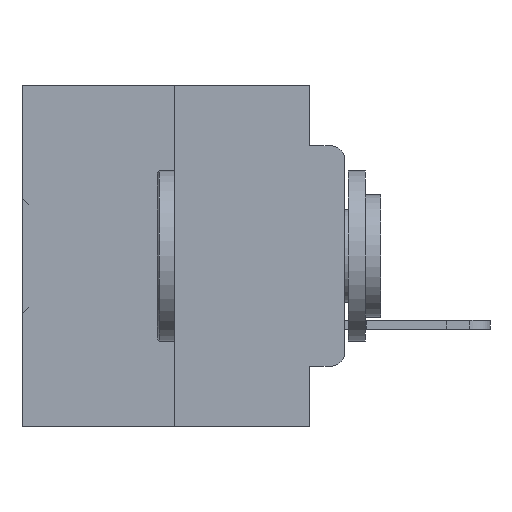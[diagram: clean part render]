
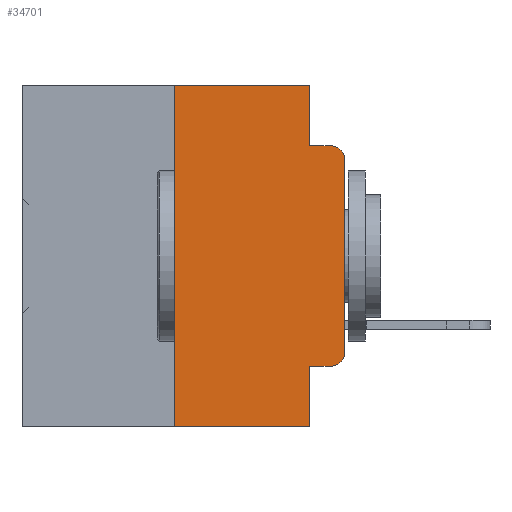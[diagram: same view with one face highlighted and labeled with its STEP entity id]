
A CAD part, left-side view. The second image highlights one B-rep face of the part: STEP entity #34701.
In plain terms, the highlighted planar face has unit normal (-1, 0, 0).
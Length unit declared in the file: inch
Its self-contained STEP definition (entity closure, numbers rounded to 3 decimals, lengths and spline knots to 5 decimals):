
#15 = CARTESIAN_POINT ( 'NONE',  ( 0., 0.051, 0. ) ) ;
#443 = EDGE_CURVE ( 'NONE', #1625, #14558, #28844, .T. ) ;
#584 = CARTESIAN_POINT ( 'NONE',  ( 0., 0.25, -0.5 ) ) ;
#693 = EDGE_CURVE ( 'NONE', #1318, #21653, #5347, .T. ) ;
#1136 = DIRECTION ( 'NONE',  ( 0., -1., 0. ) ) ;
#1315 = DIRECTION ( 'NONE',  ( 0., -1., 0. ) ) ;
#1318 = VERTEX_POINT ( 'NONE', #35348 ) ;
#1625 = VERTEX_POINT ( 'NONE', #584 ) ;
#2492 = AXIS2_PLACEMENT_3D ( 'NONE', #33372, #22013, #4564 ) ;
#2989 = CARTESIAN_POINT ( 'NONE',  ( 0., 0.051, -0.0885 ) ) ;
#3090 = VERTEX_POINT ( 'NONE', #33806 ) ;
#4260 = CARTESIAN_POINT ( 'NONE',  ( 0., 0.02, -0.0885 ) ) ;
#4564 = DIRECTION ( 'NONE',  ( 0., 0., -1. ) ) ;
#4862 = EDGE_LOOP ( 'NONE', ( #25022, #6470, #13825, #23275, #28598, #12962, #29947, #21050, #22870, #6101 ) ) ;
#5112 = DIRECTION ( 'NONE',  ( 0., 0., 1. ) ) ;
#5347 = CIRCLE ( 'NONE', #18586, 0.02 ) ;
#5638 = VERTEX_POINT ( 'NONE', #25015 ) ;
#5661 = VECTOR ( 'NONE', #1315, 39.37008 ) ;
#6101 = ORIENTED_EDGE ( 'NONE', *, *, #693, .T. ) ;
#6470 = ORIENTED_EDGE ( 'NONE', *, *, #9914, .T. ) ;
#6495 = DIRECTION ( 'NONE',  ( -1., 0., 0. ) ) ;
#6536 = VERTEX_POINT ( 'NONE', #15 ) ;
#7544 = AXIS2_PLACEMENT_3D ( 'NONE', #23849, #6495, #26697 ) ;
#8058 = CARTESIAN_POINT ( 'NONE',  ( 0., 0., 0. ) ) ;
#9769 = CARTESIAN_POINT ( 'NONE',  ( 0., 0.051, -0.4115 ) ) ;
#9914 = EDGE_CURVE ( 'NONE', #3090, #18468, #18216, .T. ) ;
#10889 = VECTOR ( 'NONE', #26927, 39.37008 ) ;
#11349 = EDGE_CURVE ( 'NONE', #11731, #26346, #11778, .T. ) ;
#11731 = VERTEX_POINT ( 'NONE', #26685 ) ;
#11777 = LINE ( 'NONE', #9769, #10889 ) ;
#11778 = LINE ( 'NONE', #13559, #26139 ) ;
#12584 = EDGE_CURVE ( 'NONE', #14558, #6536, #21103, .T. ) ;
#12962 = ORIENTED_EDGE ( 'NONE', *, *, #443, .F. ) ;
#13559 = CARTESIAN_POINT ( 'NONE',  ( 0., 0.051, 0. ) ) ;
#13646 = DIRECTION ( 'NONE',  ( 0., 0., 1. ) ) ;
#13825 = ORIENTED_EDGE ( 'NONE', *, *, #31699, .F. ) ;
#14158 = VECTOR ( 'NONE', #1136, 39.37008 ) ;
#14558 = VERTEX_POINT ( 'NONE', #20987 ) ;
#15344 = CARTESIAN_POINT ( 'NONE',  ( 0., 0.25, 0. ) ) ;
#18216 = CIRCLE ( 'NONE', #7544, 0.02 ) ;
#18345 = EDGE_CURVE ( 'NONE', #6536, #5638, #32594, .T. ) ;
#18468 = VERTEX_POINT ( 'NONE', #4260 ) ;
#18586 = AXIS2_PLACEMENT_3D ( 'NONE', #32917, #37445, #35901 ) ;
#18597 = CARTESIAN_POINT ( 'NONE',  ( 0., 0.051, -0.5 ) ) ;
#19162 = PLANE ( 'NONE',  #2492 ) ;
#20987 = CARTESIAN_POINT ( 'NONE',  ( 0., 0.25, 0. ) ) ;
#21050 = ORIENTED_EDGE ( 'NONE', *, *, #11349, .F. ) ;
#21103 = LINE ( 'NONE', #36110, #5661 ) ;
#21259 = VECTOR ( 'NONE', #13646, 39.37008 ) ;
#21653 = VERTEX_POINT ( 'NONE', #29732 ) ;
#21979 = VECTOR ( 'NONE', #5112, 39.37008 ) ;
#22013 = DIRECTION ( 'NONE',  ( 1., 0., 0. ) ) ;
#22870 = ORIENTED_EDGE ( 'NONE', *, *, #33903, .T. ) ;
#23275 = ORIENTED_EDGE ( 'NONE', *, *, #18345, .F. ) ;
#23849 = CARTESIAN_POINT ( 'NONE',  ( 0., 0.02, -0.1085 ) ) ;
#25015 = CARTESIAN_POINT ( 'NONE',  ( 0., 0.051, -0.0885 ) ) ;
#25022 = ORIENTED_EDGE ( 'NONE', *, *, #27209, .T. ) ;
#25061 = VECTOR ( 'NONE', #32677, 39.37008 ) ;
#25644 = VECTOR ( 'NONE', #26288, 39.37008 ) ;
#25928 = EDGE_CURVE ( 'NONE', #1625, #26346, #36972, .T. ) ;
#26139 = VECTOR ( 'NONE', #33707, 39.37008 ) ;
#26288 = DIRECTION ( 'NONE',  ( 0., -1., 0. ) ) ;
#26346 = VERTEX_POINT ( 'NONE', #18597 ) ;
#26526 = LINE ( 'NONE', #2989, #25644 ) ;
#26685 = CARTESIAN_POINT ( 'NONE',  ( 0., 0.051, -0.4115 ) ) ;
#26697 = DIRECTION ( 'NONE',  ( 0., 0., -1. ) ) ;
#26927 = DIRECTION ( 'NONE',  ( 0., -1., 0. ) ) ;
#27209 = EDGE_CURVE ( 'NONE', #21653, #3090, #37148, .T. ) ;
#28598 = ORIENTED_EDGE ( 'NONE', *, *, #12584, .F. ) ;
#28844 = LINE ( 'NONE', #15344, #21259 ) ;
#29732 = CARTESIAN_POINT ( 'NONE',  ( 0., 0., -0.3915 ) ) ;
#29820 = CARTESIAN_POINT ( 'NONE',  ( 0., 0.051, 0. ) ) ;
#29947 = ORIENTED_EDGE ( 'NONE', *, *, #25928, .T. ) ;
#31699 = EDGE_CURVE ( 'NONE', #5638, #18468, #26526, .T. ) ;
#32594 = LINE ( 'NONE', #29820, #25061 ) ;
#32677 = DIRECTION ( 'NONE',  ( 0., 0., -1. ) ) ;
#32917 = CARTESIAN_POINT ( 'NONE',  ( 0., 0.02, -0.3915 ) ) ;
#33372 = CARTESIAN_POINT ( 'NONE',  ( 0., 0.473, 0. ) ) ;
#33707 = DIRECTION ( 'NONE',  ( 0., 0., -1. ) ) ;
#33806 = CARTESIAN_POINT ( 'NONE',  ( 0., 0., -0.1085 ) ) ;
#33903 = EDGE_CURVE ( 'NONE', #11731, #1318, #11777, .T. ) ;
#34701 = ADVANCED_FACE ( 'NONE', ( #35464 ), #19162, .F. ) ;
#35348 = CARTESIAN_POINT ( 'NONE',  ( 0., 0.02, -0.4115 ) ) ;
#35464 = FACE_OUTER_BOUND ( 'NONE', #4862, .T. ) ;
#35901 = DIRECTION ( 'NONE',  ( 0., 0., -1. ) ) ;
#36094 = CARTESIAN_POINT ( 'NONE',  ( 0., 0.473, -0.5 ) ) ;
#36110 = CARTESIAN_POINT ( 'NONE',  ( 0., 0.473, 0. ) ) ;
#36972 = LINE ( 'NONE', #36094, #14158 ) ;
#37148 = LINE ( 'NONE', #8058, #21979 ) ;
#37445 = DIRECTION ( 'NONE',  ( -1., 0., 0. ) ) ;
